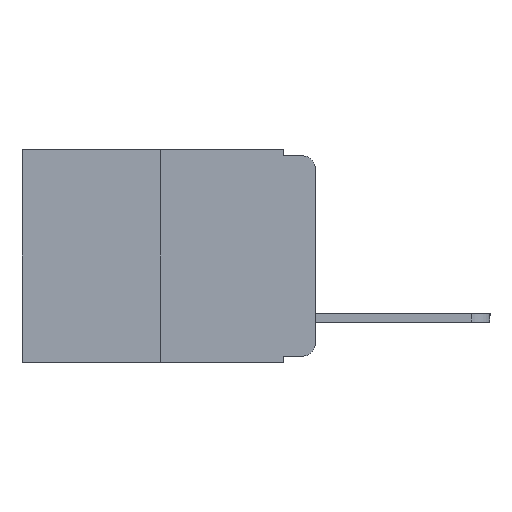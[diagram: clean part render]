
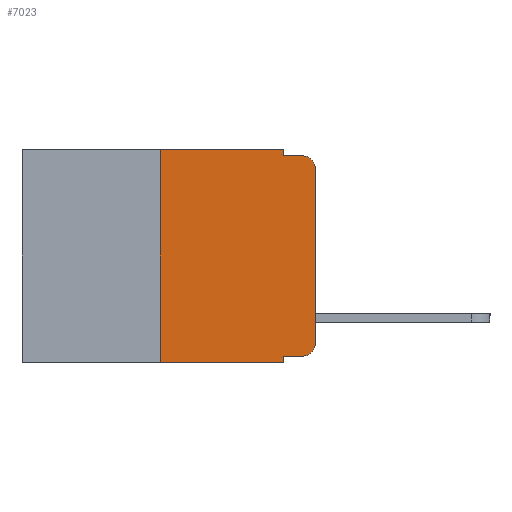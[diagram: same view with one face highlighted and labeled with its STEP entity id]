
A CAD part, left-side view. The second image highlights one B-rep face of the part: STEP entity #7023.
In plain terms, the highlighted planar face has unit normal (-1, 0, 0).
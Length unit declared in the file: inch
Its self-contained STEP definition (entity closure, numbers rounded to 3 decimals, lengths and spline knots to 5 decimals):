
#705 = VECTOR ( 'NONE', #1262, 39.37008 ) ;
#710 = VERTEX_POINT ( 'NONE', #10473 ) ;
#1137 = DIRECTION ( 'NONE',  ( 0., -1., 0. ) ) ;
#1262 = DIRECTION ( 'NONE',  ( 0., -1., 0. ) ) ;
#1278 = CARTESIAN_POINT ( 'NONE',  ( 0., 0., -0.03 ) ) ;
#1304 = ORIENTED_EDGE ( 'NONE', *, *, #16230, .T. ) ;
#1525 = CARTESIAN_POINT ( 'NONE',  ( 0., 0.25, 0. ) ) ;
#1774 = DIRECTION ( 'NONE',  ( -1., 0., 0. ) ) ;
#1872 = EDGE_CURVE ( 'NONE', #7560, #2048, #4471, .T. ) ;
#2048 = VERTEX_POINT ( 'NONE', #1525 ) ;
#2300 = VERTEX_POINT ( 'NONE', #11745 ) ;
#2443 = DIRECTION ( 'NONE',  ( 0., 0., -1. ) ) ;
#2899 = LINE ( 'NONE', #10038, #10191 ) ;
#3094 = ORIENTED_EDGE ( 'NONE', *, *, #13090, .T. ) ;
#3595 = LINE ( 'NONE', #16619, #14555 ) ;
#3716 = VECTOR ( 'NONE', #14667, 39.37008 ) ;
#3814 = CARTESIAN_POINT ( 'NONE',  ( 0., 0., -0.313 ) ) ;
#4049 = ORIENTED_EDGE ( 'NONE', *, *, #1872, .F. ) ;
#4222 = CARTESIAN_POINT ( 'NONE',  ( 0., 0.051, -0.333 ) ) ;
#4224 = CARTESIAN_POINT ( 'NONE',  ( 0., 0.02, -0.313 ) ) ;
#4411 = CARTESIAN_POINT ( 'NONE',  ( 0., 0.051, -0.01 ) ) ;
#4417 = FACE_OUTER_BOUND ( 'NONE', #17630, .T. ) ;
#4471 = LINE ( 'NONE', #8051, #14944 ) ;
#4707 = CARTESIAN_POINT ( 'NONE',  ( 0., 0.473, -0.343 ) ) ;
#4913 = VERTEX_POINT ( 'NONE', #18067 ) ;
#5021 = VERTEX_POINT ( 'NONE', #1278 ) ;
#5057 = ORIENTED_EDGE ( 'NONE', *, *, #18516, .F. ) ;
#5199 = DIRECTION ( 'NONE',  ( 0., 0., 1. ) ) ;
#5242 = DIRECTION ( 'NONE',  ( 1., 0., 0. ) ) ;
#5742 = DIRECTION ( 'NONE',  ( 0., 0., -1. ) ) ;
#5883 = VERTEX_POINT ( 'NONE', #10023 ) ;
#5964 = VECTOR ( 'NONE', #8263, 39.37008 ) ;
#6359 = VERTEX_POINT ( 'NONE', #3814 ) ;
#6505 = AXIS2_PLACEMENT_3D ( 'NONE', #10605, #1774, #12019 ) ;
#6599 = VERTEX_POINT ( 'NONE', #18204 ) ;
#7023 = ADVANCED_FACE ( 'NONE', ( #4417 ), #10927, .F. ) ;
#7560 = VERTEX_POINT ( 'NONE', #13552 ) ;
#7660 = LINE ( 'NONE', #4707, #11801 ) ;
#7885 = VERTEX_POINT ( 'NONE', #4222 ) ;
#7971 = EDGE_CURVE ( 'NONE', #2300, #710, #12463, .T. ) ;
#8051 = CARTESIAN_POINT ( 'NONE',  ( 0., 0.25, 0. ) ) ;
#8263 = DIRECTION ( 'NONE',  ( 0., 0., 1. ) ) ;
#8307 = CIRCLE ( 'NONE', #6505, 0.02 ) ;
#8417 = ORIENTED_EDGE ( 'NONE', *, *, #14134, .T. ) ;
#8865 = LINE ( 'NONE', #17868, #5964 ) ;
#8993 = AXIS2_PLACEMENT_3D ( 'NONE', #4224, #14213, #5742 ) ;
#9365 = EDGE_CURVE ( 'NONE', #6599, #2300, #16448, .T. ) ;
#10023 = CARTESIAN_POINT ( 'NONE',  ( 0., 0.02, -0.333 ) ) ;
#10038 = CARTESIAN_POINT ( 'NONE',  ( 0., 0.473, 0. ) ) ;
#10191 = VECTOR ( 'NONE', #1137, 39.37008 ) ;
#10473 = CARTESIAN_POINT ( 'NONE',  ( 0., 0.02, -0.01 ) ) ;
#10605 = CARTESIAN_POINT ( 'NONE',  ( 0., 0.02, -0.03 ) ) ;
#10808 = CARTESIAN_POINT ( 'NONE',  ( 0., 0.051, 0. ) ) ;
#10872 = EDGE_CURVE ( 'NONE', #6359, #5021, #8865, .T. ) ;
#10874 = CARTESIAN_POINT ( 'NONE',  ( 0., 0.473, 0. ) ) ;
#10913 = EDGE_CURVE ( 'NONE', #7885, #4913, #3595, .T. ) ;
#10927 = PLANE ( 'NONE',  #13504 ) ;
#11248 = ORIENTED_EDGE ( 'NONE', *, *, #13752, .T. ) ;
#11377 = LINE ( 'NONE', #11857, #3716 ) ;
#11745 = CARTESIAN_POINT ( 'NONE',  ( 0., 0.051, -0.01 ) ) ;
#11801 = VECTOR ( 'NONE', #13262, 39.37008 ) ;
#11857 = CARTESIAN_POINT ( 'NONE',  ( 0., 0.051, -0.333 ) ) ;
#11873 = ORIENTED_EDGE ( 'NONE', *, *, #7971, .F. ) ;
#12019 = DIRECTION ( 'NONE',  ( 0., 0., -1. ) ) ;
#12463 = LINE ( 'NONE', #4411, #705 ) ;
#12846 = VECTOR ( 'NONE', #17618, 39.37008 ) ;
#13090 = EDGE_CURVE ( 'NONE', #7885, #5883, #11377, .T. ) ;
#13262 = DIRECTION ( 'NONE',  ( 0., -1., 0. ) ) ;
#13504 = AXIS2_PLACEMENT_3D ( 'NONE', #10874, #5242, #15142 ) ;
#13552 = CARTESIAN_POINT ( 'NONE',  ( 0., 0.25, -0.343 ) ) ;
#13735 = ORIENTED_EDGE ( 'NONE', *, *, #10913, .F. ) ;
#13752 = EDGE_CURVE ( 'NONE', #5021, #710, #8307, .T. ) ;
#14134 = EDGE_CURVE ( 'NONE', #5883, #6359, #16897, .T. ) ;
#14213 = DIRECTION ( 'NONE',  ( -1., 0., 0. ) ) ;
#14555 = VECTOR ( 'NONE', #2443, 39.37008 ) ;
#14667 = DIRECTION ( 'NONE',  ( 0., -1., 0. ) ) ;
#14944 = VECTOR ( 'NONE', #5199, 39.37008 ) ;
#15142 = DIRECTION ( 'NONE',  ( 0., 0., -1. ) ) ;
#16230 = EDGE_CURVE ( 'NONE', #7560, #4913, #7660, .T. ) ;
#16377 = ORIENTED_EDGE ( 'NONE', *, *, #9365, .F. ) ;
#16448 = LINE ( 'NONE', #10808, #12846 ) ;
#16619 = CARTESIAN_POINT ( 'NONE',  ( 0., 0.051, 0. ) ) ;
#16897 = CIRCLE ( 'NONE', #8993, 0.02 ) ;
#17194 = ORIENTED_EDGE ( 'NONE', *, *, #10872, .T. ) ;
#17618 = DIRECTION ( 'NONE',  ( 0., 0., -1. ) ) ;
#17630 = EDGE_LOOP ( 'NONE', ( #17194, #11248, #11873, #16377, #5057, #4049, #1304, #13735, #3094, #8417 ) ) ;
#17868 = CARTESIAN_POINT ( 'NONE',  ( 0., 0., 0. ) ) ;
#18067 = CARTESIAN_POINT ( 'NONE',  ( 0., 0.051, -0.343 ) ) ;
#18204 = CARTESIAN_POINT ( 'NONE',  ( 0., 0.051, 0. ) ) ;
#18516 = EDGE_CURVE ( 'NONE', #2048, #6599, #2899, .T. ) ;
